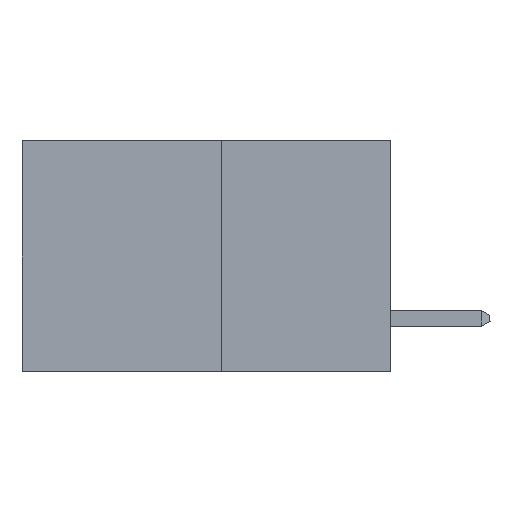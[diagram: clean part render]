
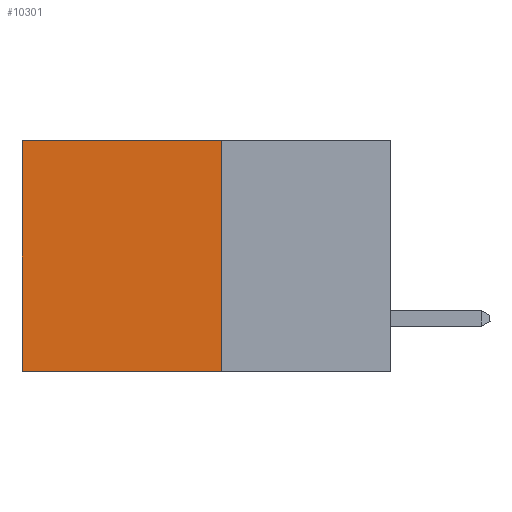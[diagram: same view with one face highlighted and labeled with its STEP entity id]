
A CAD part, left-side view. The second image highlights one B-rep face of the part: STEP entity #10301.
In plain terms, the highlighted planar face has unit normal (-1, 0, 0).
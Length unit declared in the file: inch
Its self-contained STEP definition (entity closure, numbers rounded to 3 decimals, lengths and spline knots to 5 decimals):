
#175 = VECTOR ( 'NONE', #16664, 39.37008 ) ;
#753 = EDGE_CURVE ( 'NONE', #16663, #14074, #16950, .T. ) ;
#1560 = CARTESIAN_POINT ( 'NONE',  ( 0.277, 0.59, -0.37 ) ) ;
#1878 = VERTEX_POINT ( 'NONE', #1560 ) ;
#3643 = CARTESIAN_POINT ( 'NONE',  ( 0.277, 0.59, -0.37 ) ) ;
#3718 = VERTEX_POINT ( 'NONE', #15549 ) ;
#3988 = PLANE ( 'NONE',  #7250 ) ;
#4642 = EDGE_LOOP ( 'NONE', ( #8999, #5844, #16755, #8932 ) ) ;
#5350 = DIRECTION ( 'NONE',  ( 1., 0., 0. ) ) ;
#5615 = CARTESIAN_POINT ( 'NONE',  ( 0.277, 0.59, 0. ) ) ;
#5721 = CARTESIAN_POINT ( 'NONE',  ( 0.277, 0.27, 0. ) ) ;
#5844 = ORIENTED_EDGE ( 'NONE', *, *, #15813, .F. ) ;
#6143 = CARTESIAN_POINT ( 'NONE',  ( 0.277, 0.27, -0.37 ) ) ;
#7250 = AXIS2_PLACEMENT_3D ( 'NONE', #13307, #5350, #14597 ) ;
#7775 = VECTOR ( 'NONE', #12027, 39.37008 ) ;
#8932 = ORIENTED_EDGE ( 'NONE', *, *, #753, .T. ) ;
#8999 = ORIENTED_EDGE ( 'NONE', *, *, #11997, .T. ) ;
#10050 = VECTOR ( 'NONE', #13215, 39.37008 ) ;
#10301 = ADVANCED_FACE ( 'NONE', ( #12944 ), #3988, .F. ) ;
#10349 = DIRECTION ( 'NONE',  ( 0., 0., -1. ) ) ;
#10671 = CARTESIAN_POINT ( 'NONE',  ( 0.277, 0.27, -0.37 ) ) ;
#11749 = LINE ( 'NONE', #10671, #7775 ) ;
#11997 = EDGE_CURVE ( 'NONE', #14074, #1878, #16519, .T. ) ;
#12027 = DIRECTION ( 'NONE',  ( 0., 1., 0. ) ) ;
#12944 = FACE_OUTER_BOUND ( 'NONE', #4642, .T. ) ;
#13107 = CARTESIAN_POINT ( 'NONE',  ( 0.277, 0.27, 0. ) ) ;
#13215 = DIRECTION ( 'NONE',  ( 0., 1., 0. ) ) ;
#13307 = CARTESIAN_POINT ( 'NONE',  ( 0.277, 0.27, -0.37 ) ) ;
#14074 = VERTEX_POINT ( 'NONE', #5615 ) ;
#14295 = LINE ( 'NONE', #6143, #175 ) ;
#14597 = DIRECTION ( 'NONE',  ( 0., 0., -1. ) ) ;
#15549 = CARTESIAN_POINT ( 'NONE',  ( 0.277, 0.27, -0.37 ) ) ;
#15813 = EDGE_CURVE ( 'NONE', #3718, #1878, #11749, .T. ) ;
#16111 = VECTOR ( 'NONE', #10349, 39.37008 ) ;
#16519 = LINE ( 'NONE', #3643, #16111 ) ;
#16663 = VERTEX_POINT ( 'NONE', #5721 ) ;
#16664 = DIRECTION ( 'NONE',  ( 0., 0., -1. ) ) ;
#16755 = ORIENTED_EDGE ( 'NONE', *, *, #16794, .F. ) ;
#16794 = EDGE_CURVE ( 'NONE', #16663, #3718, #14295, .T. ) ;
#16950 = LINE ( 'NONE', #13107, #10050 ) ;
